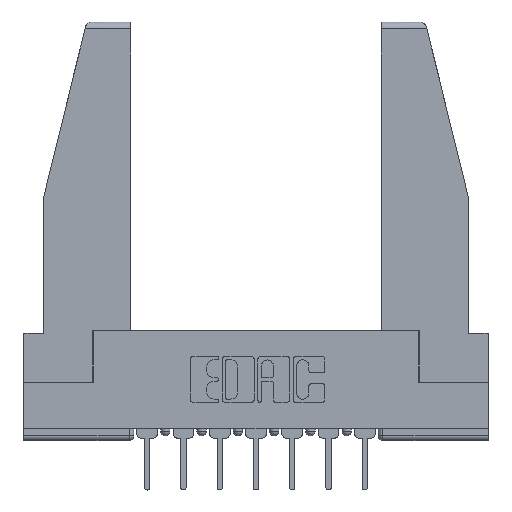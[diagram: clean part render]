
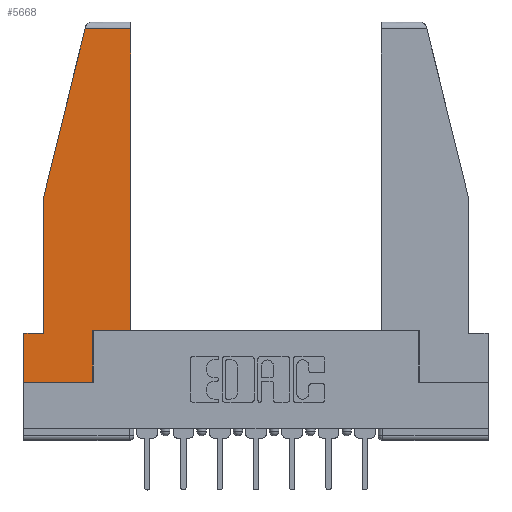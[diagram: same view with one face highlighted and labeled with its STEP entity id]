
A CAD part, top view. The second image highlights one B-rep face of the part: STEP entity #5668.
In plain terms, the highlighted planar face has unit normal (0, 0, 1).
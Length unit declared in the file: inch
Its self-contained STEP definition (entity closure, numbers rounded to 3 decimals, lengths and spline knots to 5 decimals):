
#4 = ORIENTED_EDGE ( 'NONE', *, *, #8072, .T. ) ;
#354 = AXIS2_PLACEMENT_3D ( 'NONE', #11461, #6651, #9544 ) ;
#590 = ORIENTED_EDGE ( 'NONE', *, *, #8455, .T. ) ;
#828 = DIRECTION ( 'NONE',  ( -1., 0., 0. ) ) ;
#875 = FACE_OUTER_BOUND ( 'NONE', #2231, .T. ) ;
#898 = CARTESIAN_POINT ( 'NONE',  ( 0.297, 0.223, 0. ) ) ;
#988 = CARTESIAN_POINT ( 'NONE',  ( 0., 0., 0. ) ) ;
#1035 = CARTESIAN_POINT ( 'NONE',  ( 0.297, 0., 0. ) ) ;
#1045 = VECTOR ( 'NONE', #7848, 39.37008 ) ;
#1485 = DIRECTION ( 'NONE',  ( 0., -1., 0. ) ) ;
#1635 = VECTOR ( 'NONE', #4476, 39.37008 ) ;
#1806 = ORIENTED_EDGE ( 'NONE', *, *, #6350, .T. ) ;
#2231 = EDGE_LOOP ( 'NONE', ( #9127, #11914, #4000, #1806, #4, #4819, #10130, #2422, #590 ) ) ;
#2286 = CARTESIAN_POINT ( 'NONE',  ( 0.086, 0.21, 0. ) ) ;
#2422 = ORIENTED_EDGE ( 'NONE', *, *, #5523, .T. ) ;
#2961 = VECTOR ( 'NONE', #8677, 39.37008 ) ;
#3009 = CARTESIAN_POINT ( 'NONE',  ( 0.271, 1.55, 0. ) ) ;
#3064 = CARTESIAN_POINT ( 'NONE',  ( 0.086, 0.8, 0. ) ) ;
#3097 = CARTESIAN_POINT ( 'NONE',  ( 0.297, 0.223, 0. ) ) ;
#3143 = LINE ( 'NONE', #8669, #11481 ) ;
#3315 = CARTESIAN_POINT ( 'NONE',  ( 0.2636, 1.52, 0. ) ) ;
#3462 = VERTEX_POINT ( 'NONE', #1035 ) ;
#3785 = VERTEX_POINT ( 'NONE', #2286 ) ;
#4000 = ORIENTED_EDGE ( 'NONE', *, *, #11834, .T. ) ;
#4115 = EDGE_CURVE ( 'NONE', #5931, #3462, #8270, .T. ) ;
#4191 = LINE ( 'NONE', #9683, #2961 ) ;
#4476 = DIRECTION ( 'NONE',  ( 0., 1., 0. ) ) ;
#4819 = ORIENTED_EDGE ( 'NONE', *, *, #6104, .T. ) ;
#4993 = CARTESIAN_POINT ( 'NONE',  ( 0.461, 0.223, 0. ) ) ;
#5013 = VECTOR ( 'NONE', #5522, 39.37008 ) ;
#5522 = DIRECTION ( 'NONE',  ( -1., 0., 0. ) ) ;
#5523 = EDGE_CURVE ( 'NONE', #3462, #7102, #5803, .T. ) ;
#5662 = CARTESIAN_POINT ( 'NONE',  ( 0.461, 1.52, 0. ) ) ;
#5668 = ADVANCED_FACE ( 'NONE', ( #875 ), #10453, .T. ) ;
#5779 = CARTESIAN_POINT ( 'NONE',  ( 0., 0.21, 0. ) ) ;
#5803 = LINE ( 'NONE', #9421, #1635 ) ;
#5839 = VERTEX_POINT ( 'NONE', #10839 ) ;
#5931 = VERTEX_POINT ( 'NONE', #9473 ) ;
#6104 = EDGE_CURVE ( 'NONE', #5839, #5931, #6451, .T. ) ;
#6167 = VERTEX_POINT ( 'NONE', #4993 ) ;
#6350 = EDGE_CURVE ( 'NONE', #11341, #3785, #7807, .T. ) ;
#6451 = LINE ( 'NONE', #5779, #1045 ) ;
#6651 = DIRECTION ( 'NONE',  ( 0., 0., 1. ) ) ;
#6894 = VECTOR ( 'NONE', #10592, 39.37008 ) ;
#7102 = VERTEX_POINT ( 'NONE', #898 ) ;
#7271 = CARTESIAN_POINT ( 'NONE',  ( 0.086, 0.8, 0. ) ) ;
#7640 = VERTEX_POINT ( 'NONE', #5662 ) ;
#7807 = LINE ( 'NONE', #7271, #11054 ) ;
#7848 = DIRECTION ( 'NONE',  ( 0., -1., 0. ) ) ;
#8063 = DIRECTION ( 'NONE',  ( 1., 0., 0. ) ) ;
#8072 = EDGE_CURVE ( 'NONE', #3785, #5839, #11013, .T. ) ;
#8270 = LINE ( 'NONE', #988, #6894 ) ;
#8292 = CARTESIAN_POINT ( 'NONE',  ( 0., 0.21, 0. ) ) ;
#8455 = EDGE_CURVE ( 'NONE', #7102, #6167, #12554, .T. ) ;
#8669 = CARTESIAN_POINT ( 'NONE',  ( 0., 1.52, 0. ) ) ;
#8677 = DIRECTION ( 'NONE',  ( 0., 1., 0. ) ) ;
#8856 = EDGE_CURVE ( 'NONE', #7640, #12567, #3143, .T. ) ;
#9127 = ORIENTED_EDGE ( 'NONE', *, *, #9950, .T. ) ;
#9421 = CARTESIAN_POINT ( 'NONE',  ( 0.297, 0., 0. ) ) ;
#9473 = CARTESIAN_POINT ( 'NONE',  ( 0., 0., 0. ) ) ;
#9544 = DIRECTION ( 'NONE',  ( 1., 0., 0. ) ) ;
#9683 = CARTESIAN_POINT ( 'NONE',  ( 0.461, 0.223, 0. ) ) ;
#9816 = DIRECTION ( 'NONE',  ( -0.239, -0.971, 0. ) ) ;
#9950 = EDGE_CURVE ( 'NONE', #6167, #7640, #4191, .T. ) ;
#10130 = ORIENTED_EDGE ( 'NONE', *, *, #4115, .T. ) ;
#10453 = PLANE ( 'NONE',  #354 ) ;
#10592 = DIRECTION ( 'NONE',  ( 1., 0., 0. ) ) ;
#10839 = CARTESIAN_POINT ( 'NONE',  ( 0., 0.21, 0. ) ) ;
#11013 = LINE ( 'NONE', #8292, #5013 ) ;
#11054 = VECTOR ( 'NONE', #1485, 39.37008 ) ;
#11341 = VERTEX_POINT ( 'NONE', #3064 ) ;
#11461 = CARTESIAN_POINT ( 'NONE',  ( 0., 0., 0. ) ) ;
#11481 = VECTOR ( 'NONE', #828, 39.37008 ) ;
#11834 = EDGE_CURVE ( 'NONE', #12567, #11341, #11867, .T. ) ;
#11867 = LINE ( 'NONE', #3009, #12166 ) ;
#11914 = ORIENTED_EDGE ( 'NONE', *, *, #8856, .T. ) ;
#11936 = VECTOR ( 'NONE', #8063, 39.37008 ) ;
#12166 = VECTOR ( 'NONE', #9816, 39.37008 ) ;
#12554 = LINE ( 'NONE', #3097, #11936 ) ;
#12567 = VERTEX_POINT ( 'NONE', #3315 ) ;
